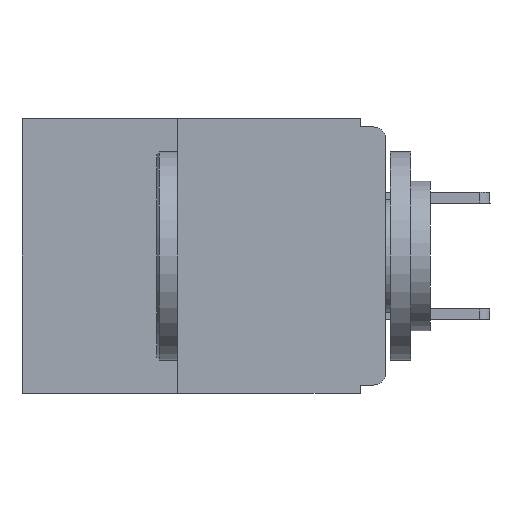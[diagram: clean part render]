
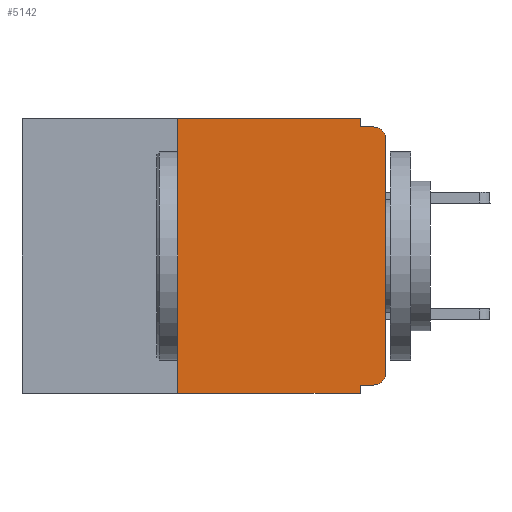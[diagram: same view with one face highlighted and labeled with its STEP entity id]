
A CAD part, left-side view. The second image highlights one B-rep face of the part: STEP entity #5142.
In plain terms, the highlighted planar face has unit normal (-1, 0, 0).
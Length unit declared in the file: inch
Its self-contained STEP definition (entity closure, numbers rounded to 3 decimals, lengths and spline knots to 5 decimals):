
#111 = ORIENTED_EDGE ( 'NONE', *, *, #4827, .F. ) ;
#221 = EDGE_CURVE ( 'NONE', #4157, #1802, #1616, .T. ) ;
#280 = CARTESIAN_POINT ( 'NONE',  ( 0., 0.015, -0.305 ) ) ;
#447 = CARTESIAN_POINT ( 'NONE',  ( 0., 0.25, -0.33 ) ) ;
#685 = FACE_OUTER_BOUND ( 'NONE', #1162, .T. ) ;
#687 = VECTOR ( 'NONE', #1909, 39.37008 ) ;
#774 = CARTESIAN_POINT ( 'NONE',  ( 0., 0.437, 0. ) ) ;
#812 = LINE ( 'NONE', #10701, #2979 ) ;
#1055 = VECTOR ( 'NONE', #9042, 39.37008 ) ;
#1162 = EDGE_LOOP ( 'NONE', ( #11951, #7770, #11403, #9762, #111, #3386, #10621, #11349, #6703, #5403 ) ) ;
#1516 = DIRECTION ( 'NONE',  ( 0., 0., 1. ) ) ;
#1616 = LINE ( 'NONE', #3470, #10268 ) ;
#1622 = CARTESIAN_POINT ( 'NONE',  ( 0., 0.031, -0.33 ) ) ;
#1802 = VERTEX_POINT ( 'NONE', #7038 ) ;
#1820 = CARTESIAN_POINT ( 'NONE',  ( 0., 0.015, -0.32 ) ) ;
#1909 = DIRECTION ( 'NONE',  ( 0., 0., 1. ) ) ;
#1976 = EDGE_CURVE ( 'NONE', #2071, #2119, #2003, .T. ) ;
#2003 = LINE ( 'NONE', #2778, #687 ) ;
#2071 = VERTEX_POINT ( 'NONE', #447 ) ;
#2079 = VERTEX_POINT ( 'NONE', #2265 ) ;
#2119 = VERTEX_POINT ( 'NONE', #8742 ) ;
#2224 = VERTEX_POINT ( 'NONE', #4717 ) ;
#2265 = CARTESIAN_POINT ( 'NONE',  ( 0., 0.015, -0.01 ) ) ;
#2455 = EDGE_CURVE ( 'NONE', #3101, #3612, #812, .T. ) ;
#2778 = CARTESIAN_POINT ( 'NONE',  ( 0., 0.25, -0.33 ) ) ;
#2950 = AXIS2_PLACEMENT_3D ( 'NONE', #11720, #5166, #6912 ) ;
#2979 = VECTOR ( 'NONE', #8966, 39.37008 ) ;
#3101 = VERTEX_POINT ( 'NONE', #8177 ) ;
#3386 = ORIENTED_EDGE ( 'NONE', *, *, #1976, .F. ) ;
#3470 = CARTESIAN_POINT ( 'NONE',  ( 0., 0., 0. ) ) ;
#3612 = VERTEX_POINT ( 'NONE', #1622 ) ;
#3667 = CARTESIAN_POINT ( 'NONE',  ( 0., 0.031, 0. ) ) ;
#3969 = DIRECTION ( 'NONE',  ( 0., -1., 0. ) ) ;
#4011 = EDGE_CURVE ( 'NONE', #5937, #2224, #9844, .T. ) ;
#4157 = VERTEX_POINT ( 'NONE', #11596 ) ;
#4320 = EDGE_CURVE ( 'NONE', #11482, #4157, #9396, .T. ) ;
#4592 = CARTESIAN_POINT ( 'NONE',  ( 0., 0., -0.01 ) ) ;
#4616 = DIRECTION ( 'NONE',  ( 0., 0., -1. ) ) ;
#4648 = DIRECTION ( 'NONE',  ( 0., -1., 0. ) ) ;
#4717 = CARTESIAN_POINT ( 'NONE',  ( 0., 0.031, -0.01 ) ) ;
#4827 = EDGE_CURVE ( 'NONE', #2119, #5937, #8231, .T. ) ;
#4898 = VECTOR ( 'NONE', #4616, 39.37008 ) ;
#5040 = DIRECTION ( 'NONE',  ( 0., 0., -1. ) ) ;
#5112 = AXIS2_PLACEMENT_3D ( 'NONE', #774, #11961, #7412 ) ;
#5142 = ADVANCED_FACE ( 'NONE', ( #685 ), #7368, .F. ) ;
#5166 = DIRECTION ( 'NONE',  ( -1., 0., 0. ) ) ;
#5403 = ORIENTED_EDGE ( 'NONE', *, *, #4320, .T. ) ;
#5431 = EDGE_CURVE ( 'NONE', #1802, #2079, #8062, .T. ) ;
#5446 = CARTESIAN_POINT ( 'NONE',  ( 0., 0.437, -0.33 ) ) ;
#5701 = EDGE_CURVE ( 'NONE', #2071, #3612, #7918, .T. ) ;
#5863 = DIRECTION ( 'NONE',  ( -1., 0., 0. ) ) ;
#5937 = VERTEX_POINT ( 'NONE', #8774 ) ;
#6703 = ORIENTED_EDGE ( 'NONE', *, *, #8446, .F. ) ;
#6912 = DIRECTION ( 'NONE',  ( 0., 0., -1. ) ) ;
#7038 = CARTESIAN_POINT ( 'NONE',  ( 0., 0., -0.025 ) ) ;
#7180 = CARTESIAN_POINT ( 'NONE',  ( 0., 0., -0.32 ) ) ;
#7368 = PLANE ( 'NONE',  #5112 ) ;
#7412 = DIRECTION ( 'NONE',  ( 0., 0., -1. ) ) ;
#7427 = LINE ( 'NONE', #7180, #1055 ) ;
#7541 = EDGE_CURVE ( 'NONE', #2224, #2079, #9303, .T. ) ;
#7770 = ORIENTED_EDGE ( 'NONE', *, *, #5431, .T. ) ;
#7918 = LINE ( 'NONE', #5446, #9070 ) ;
#8004 = VECTOR ( 'NONE', #3969, 39.37008 ) ;
#8062 = CIRCLE ( 'NONE', #2950, 0.015 ) ;
#8177 = CARTESIAN_POINT ( 'NONE',  ( 0., 0.031, -0.32 ) ) ;
#8231 = LINE ( 'NONE', #10977, #9381 ) ;
#8446 = EDGE_CURVE ( 'NONE', #11482, #3101, #7427, .T. ) ;
#8742 = CARTESIAN_POINT ( 'NONE',  ( 0., 0.25, 0. ) ) ;
#8774 = CARTESIAN_POINT ( 'NONE',  ( 0., 0.031, 0. ) ) ;
#8966 = DIRECTION ( 'NONE',  ( 0., 0., -1. ) ) ;
#9042 = DIRECTION ( 'NONE',  ( 0., 1., 0. ) ) ;
#9070 = VECTOR ( 'NONE', #4648, 39.37008 ) ;
#9303 = LINE ( 'NONE', #4592, #8004 ) ;
#9381 = VECTOR ( 'NONE', #11934, 39.37008 ) ;
#9396 = CIRCLE ( 'NONE', #9695, 0.015 ) ;
#9695 = AXIS2_PLACEMENT_3D ( 'NONE', #280, #5863, #5040 ) ;
#9762 = ORIENTED_EDGE ( 'NONE', *, *, #4011, .F. ) ;
#9844 = LINE ( 'NONE', #3667, #4898 ) ;
#10268 = VECTOR ( 'NONE', #1516, 39.37008 ) ;
#10621 = ORIENTED_EDGE ( 'NONE', *, *, #5701, .T. ) ;
#10701 = CARTESIAN_POINT ( 'NONE',  ( 0., 0.031, -0.33 ) ) ;
#10977 = CARTESIAN_POINT ( 'NONE',  ( 0., 0.437, 0. ) ) ;
#11349 = ORIENTED_EDGE ( 'NONE', *, *, #2455, .F. ) ;
#11403 = ORIENTED_EDGE ( 'NONE', *, *, #7541, .F. ) ;
#11482 = VERTEX_POINT ( 'NONE', #1820 ) ;
#11596 = CARTESIAN_POINT ( 'NONE',  ( 0., 0., -0.305 ) ) ;
#11720 = CARTESIAN_POINT ( 'NONE',  ( 0., 0.015, -0.025 ) ) ;
#11934 = DIRECTION ( 'NONE',  ( 0., -1., 0. ) ) ;
#11951 = ORIENTED_EDGE ( 'NONE', *, *, #221, .T. ) ;
#11961 = DIRECTION ( 'NONE',  ( 1., 0., 0. ) ) ;
